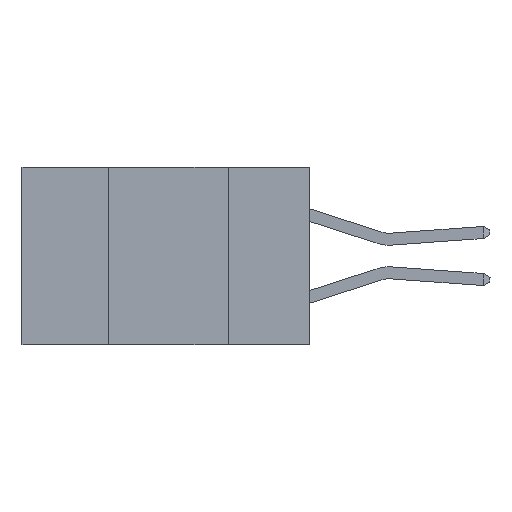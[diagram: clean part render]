
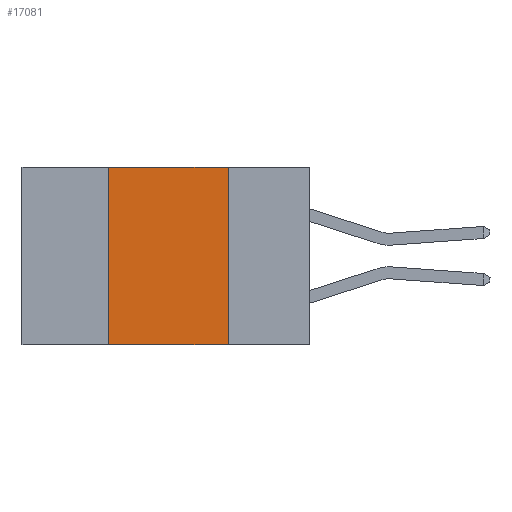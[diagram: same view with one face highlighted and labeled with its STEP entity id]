
A CAD part, left-side view. The second image highlights one B-rep face of the part: STEP entity #17081.
In plain terms, the highlighted planar face has unit normal (-1, 0, 0).
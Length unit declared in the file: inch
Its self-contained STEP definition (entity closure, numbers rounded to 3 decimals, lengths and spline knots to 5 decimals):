
#407 = VECTOR ( 'NONE', #5615, 39.37008 ) ;
#502 = EDGE_CURVE ( 'NONE', #7740, #6733, #7629, .T. ) ;
#577 = LINE ( 'NONE', #2253, #7381 ) ;
#976 = VERTEX_POINT ( 'NONE', #6785 ) ;
#1425 = EDGE_LOOP ( 'NONE', ( #6930, #14053, #7348, #10882 ) ) ;
#2253 = CARTESIAN_POINT ( 'NONE',  ( 0., 0.6, 0. ) ) ;
#4106 = CARTESIAN_POINT ( 'NONE',  ( 0., 0.6, -0.37 ) ) ;
#4320 = VECTOR ( 'NONE', #8955, 39.37008 ) ;
#5009 = DIRECTION ( 'NONE',  ( 0., -1., 0. ) ) ;
#5615 = DIRECTION ( 'NONE',  ( 0., 0., -1. ) ) ;
#6733 = VERTEX_POINT ( 'NONE', #14921 ) ;
#6785 = CARTESIAN_POINT ( 'NONE',  ( 0., 0.42, 0. ) ) ;
#6930 = ORIENTED_EDGE ( 'NONE', *, *, #502, .F. ) ;
#7348 = ORIENTED_EDGE ( 'NONE', *, *, #12579, .F. ) ;
#7381 = VECTOR ( 'NONE', #5009, 39.37008 ) ;
#7629 = LINE ( 'NONE', #12169, #407 ) ;
#7635 = LINE ( 'NONE', #4106, #14354 ) ;
#7740 = VERTEX_POINT ( 'NONE', #17154 ) ;
#7758 = CARTESIAN_POINT ( 'NONE',  ( 0., 0.6, 0. ) ) ;
#8955 = DIRECTION ( 'NONE',  ( 0., 0., 1. ) ) ;
#9110 = DIRECTION ( 'NONE',  ( 0., 0., -1. ) ) ;
#9932 = AXIS2_PLACEMENT_3D ( 'NONE', #7758, #17160, #9110 ) ;
#10685 = VERTEX_POINT ( 'NONE', #16000 ) ;
#10772 = EDGE_CURVE ( 'NONE', #10685, #6733, #7635, .T. ) ;
#10882 = ORIENTED_EDGE ( 'NONE', *, *, #10772, .T. ) ;
#12169 = CARTESIAN_POINT ( 'NONE',  ( 0., 0.17, -0.37 ) ) ;
#12579 = EDGE_CURVE ( 'NONE', #10685, #976, #14997, .T. ) ;
#14053 = ORIENTED_EDGE ( 'NONE', *, *, #14413, .F. ) ;
#14354 = VECTOR ( 'NONE', #14820, 39.37008 ) ;
#14413 = EDGE_CURVE ( 'NONE', #976, #7740, #577, .T. ) ;
#14448 = PLANE ( 'NONE',  #9932 ) ;
#14820 = DIRECTION ( 'NONE',  ( 0., -1., 0. ) ) ;
#14835 = FACE_OUTER_BOUND ( 'NONE', #1425, .T. ) ;
#14921 = CARTESIAN_POINT ( 'NONE',  ( 0., 0.17, -0.37 ) ) ;
#14997 = LINE ( 'NONE', #15654, #4320 ) ;
#15654 = CARTESIAN_POINT ( 'NONE',  ( 0., 0.42, -0.37 ) ) ;
#16000 = CARTESIAN_POINT ( 'NONE',  ( 0., 0.42, -0.37 ) ) ;
#17081 = ADVANCED_FACE ( 'NONE', ( #14835 ), #14448, .F. ) ;
#17154 = CARTESIAN_POINT ( 'NONE',  ( 0., 0.17, 0. ) ) ;
#17160 = DIRECTION ( 'NONE',  ( 1., 0., 0. ) ) ;
